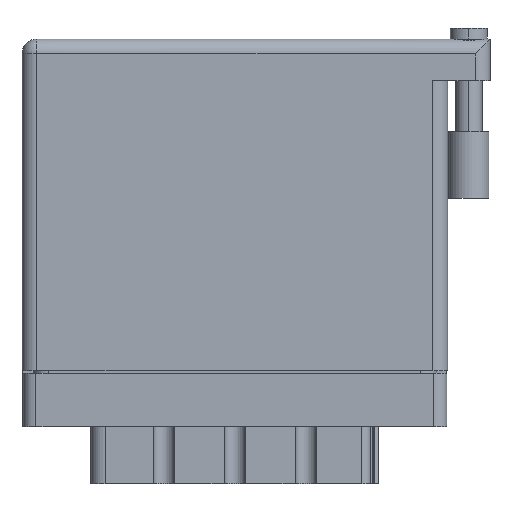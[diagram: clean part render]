
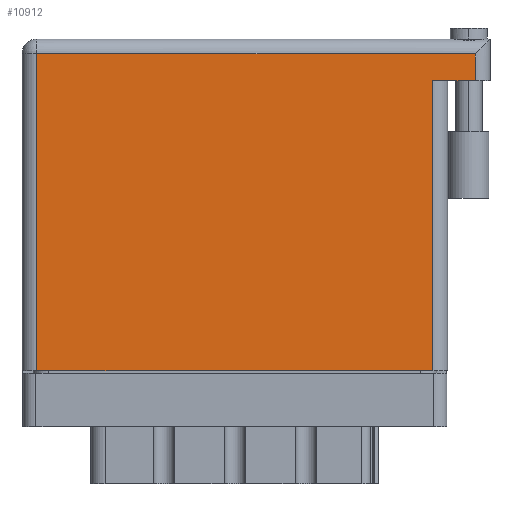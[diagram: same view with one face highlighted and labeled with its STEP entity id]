
A CAD part, front view. The second image highlights one B-rep face of the part: STEP entity #10912.
In plain terms, the highlighted face is planar.
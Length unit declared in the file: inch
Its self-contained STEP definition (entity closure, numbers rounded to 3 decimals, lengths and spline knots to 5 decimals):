
#1173 = DIRECTION ( 'NONE',  ( 1., 0., 0. ) ) ;
#2044 = EDGE_CURVE ( 'NONE', #23397, #23823, #8086, .T. ) ;
#2262 = DIRECTION ( 'NONE',  ( 0., -1., 0. ) ) ;
#2810 = ORIENTED_EDGE ( 'NONE', *, *, #31248, .T. ) ;
#3423 = LINE ( 'NONE', #31897, #16855 ) ;
#4147 = VERTEX_POINT ( 'NONE', #32679 ) ;
#4299 = CARTESIAN_POINT ( 'NONE',  ( 2.208, 1.369, 0. ) ) ;
#4858 = ORIENTED_EDGE ( 'NONE', *, *, #21706, .T. ) ;
#4870 = LINE ( 'NONE', #36346, #32550 ) ;
#5368 = ORIENTED_EDGE ( 'NONE', *, *, #2044, .F. ) ;
#5739 = EDGE_CURVE ( 'NONE', #4147, #13832, #4870, .T. ) ;
#5963 = DIRECTION ( 'NONE',  ( 0., 1., 0. ) ) ;
#6596 = DIRECTION ( 'NONE',  ( -1., 0., 0. ) ) ;
#6625 = EDGE_CURVE ( 'NONE', #32499, #4147, #3423, .T. ) ;
#6707 = LINE ( 'NONE', #29859, #19199 ) ;
#7078 = ORIENTED_EDGE ( 'NONE', *, *, #20760, .T. ) ;
#8086 = LINE ( 'NONE', #4299, #34856 ) ;
#8105 = CARTESIAN_POINT ( 'NONE',  ( 2.138, 1.496, 0. ) ) ;
#9220 = DIRECTION ( 'NONE',  ( -1., 0., 0. ) ) ;
#9242 = LINE ( 'NONE', #34271, #23112 ) ;
#10912 = ADVANCED_FACE ( 'NONE', ( #31499 ), #29285, .F. ) ;
#13832 = VERTEX_POINT ( 'NONE', #31225 ) ;
#16855 = VECTOR ( 'NONE', #9220, 39.37008 ) ;
#19199 = VECTOR ( 'NONE', #21626, 39.37008 ) ;
#20751 = CARTESIAN_POINT ( 'NONE',  ( 0., 0., 0. ) ) ;
#20760 = EDGE_CURVE ( 'NONE', #13832, #36051, #34721, .T. ) ;
#20810 = DIRECTION ( 'NONE',  ( 0., 0., -1. ) ) ;
#21626 = DIRECTION ( 'NONE',  ( 0., 1., 0. ) ) ;
#21706 = EDGE_CURVE ( 'NONE', #23397, #32499, #9242, .T. ) ;
#21767 = DIRECTION ( 'NONE',  ( -1., 0., 0. ) ) ;
#23112 = VECTOR ( 'NONE', #5963, 39.37008 ) ;
#23397 = VERTEX_POINT ( 'NONE', #36647 ) ;
#23823 = VERTEX_POINT ( 'NONE', #35510 ) ;
#25826 = EDGE_LOOP ( 'NONE', ( #7078, #2810, #5368, #4858, #34069, #29988 ) ) ;
#25893 = AXIS2_PLACEMENT_3D ( 'NONE', #29669, #20810, #6596 ) ;
#27137 = VECTOR ( 'NONE', #1173, 39.37008 ) ;
#29285 = PLANE ( 'NONE',  #25893 ) ;
#29593 = CARTESIAN_POINT ( 'NONE',  ( 1.938, 0., 0. ) ) ;
#29669 = CARTESIAN_POINT ( 'NONE',  ( 0., 1.566, 0. ) ) ;
#29859 = CARTESIAN_POINT ( 'NONE',  ( 1.938, 1.369, 0. ) ) ;
#29988 = ORIENTED_EDGE ( 'NONE', *, *, #5739, .T. ) ;
#31225 = CARTESIAN_POINT ( 'NONE',  ( 0.07, 0., 0. ) ) ;
#31248 = EDGE_CURVE ( 'NONE', #36051, #23823, #6707, .T. ) ;
#31499 = FACE_OUTER_BOUND ( 'NONE', #25826, .T. ) ;
#31897 = CARTESIAN_POINT ( 'NONE',  ( 0., 1.496, 0. ) ) ;
#32499 = VERTEX_POINT ( 'NONE', #8105 ) ;
#32550 = VECTOR ( 'NONE', #2262, 39.37008 ) ;
#32679 = CARTESIAN_POINT ( 'NONE',  ( 0.07, 1.496, 0. ) ) ;
#34069 = ORIENTED_EDGE ( 'NONE', *, *, #6625, .T. ) ;
#34271 = CARTESIAN_POINT ( 'NONE',  ( 2.138, 1.566, 0. ) ) ;
#34721 = LINE ( 'NONE', #20751, #27137 ) ;
#34856 = VECTOR ( 'NONE', #21767, 39.37008 ) ;
#35510 = CARTESIAN_POINT ( 'NONE',  ( 1.938, 1.369, 0. ) ) ;
#36051 = VERTEX_POINT ( 'NONE', #29593 ) ;
#36346 = CARTESIAN_POINT ( 'NONE',  ( 0.07, 0., 0. ) ) ;
#36647 = CARTESIAN_POINT ( 'NONE',  ( 2.138, 1.369, 0. ) ) ;
